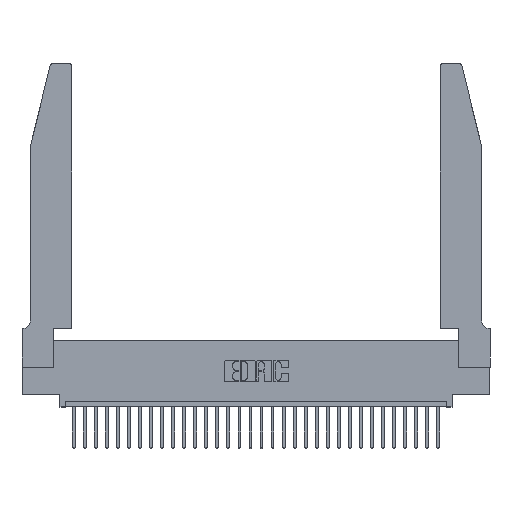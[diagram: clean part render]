
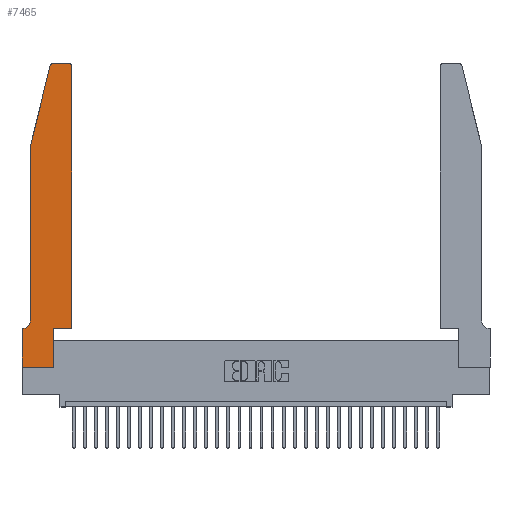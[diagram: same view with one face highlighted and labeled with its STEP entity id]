
A CAD part, top view. The second image highlights one B-rep face of the part: STEP entity #7465.
In plain terms, the highlighted planar face has unit normal (0, 0, 1).
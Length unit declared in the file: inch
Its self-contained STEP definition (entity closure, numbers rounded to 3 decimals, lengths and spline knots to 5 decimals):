
#717 = DIRECTION ( 'NONE',  ( -1., 0., 0. ) ) ;
#1285 = VECTOR ( 'NONE', #17615, 39.37008 ) ;
#1387 = ORIENTED_EDGE ( 'NONE', *, *, #26186, .T. ) ;
#1415 = CARTESIAN_POINT ( 'NONE',  ( 0., 0.35, 0.37 ) ) ;
#1495 = VERTEX_POINT ( 'NONE', #10149 ) ;
#1632 = VECTOR ( 'NONE', #23176, 39.37008 ) ;
#2771 = CARTESIAN_POINT ( 'NONE',  ( 0.2865, 0., 0.37 ) ) ;
#3564 = EDGE_LOOP ( 'NONE', ( #24043, #13470, #21757, #31179, #27198, #29213, #1387, #7926, #9912, #20818, #12689, #25088 ) ) ;
#4615 = CARTESIAN_POINT ( 'NONE',  ( 0.284, 2.72, 0.37 ) ) ;
#4989 = VERTEX_POINT ( 'NONE', #22720 ) ;
#5732 = CARTESIAN_POINT ( 'NONE',  ( 0.4205, 2.75, 0.37 ) ) ;
#5769 = CARTESIAN_POINT ( 'NONE',  ( 0.0755, 0.35, 0.37 ) ) ;
#5818 = CARTESIAN_POINT ( 'NONE',  ( 0.0755, 2., 0.37 ) ) ;
#7255 = DIRECTION ( 'NONE',  ( 1., 0., 0. ) ) ;
#7465 = ADVANCED_FACE ( 'NONE', ( #26915 ), #8958, .T. ) ;
#7489 = DIRECTION ( 'NONE',  ( 1., 0., 0. ) ) ;
#7926 = ORIENTED_EDGE ( 'NONE', *, *, #8728, .T. ) ;
#8214 = CARTESIAN_POINT ( 'NONE',  ( 0.0055, 0.35, 0.37 ) ) ;
#8228 = CARTESIAN_POINT ( 'NONE',  ( 0.4505, 0.35, 0.37 ) ) ;
#8425 = CIRCLE ( 'NONE', #11938, 0.03 ) ;
#8593 = VERTEX_POINT ( 'NONE', #23899 ) ;
#8728 = EDGE_CURVE ( 'NONE', #17757, #23434, #14239, .T. ) ;
#8958 = PLANE ( 'NONE',  #11243 ) ;
#9167 = DIRECTION ( 'NONE',  ( 0., 0., 1. ) ) ;
#9337 = VERTEX_POINT ( 'NONE', #5732 ) ;
#9739 = EDGE_CURVE ( 'NONE', #4989, #26305, #13138, .T. ) ;
#9912 = ORIENTED_EDGE ( 'NONE', *, *, #13290, .T. ) ;
#10149 = CARTESIAN_POINT ( 'NONE',  ( 0.2865, 0.35, 0.37 ) ) ;
#10569 = CIRCLE ( 'NONE', #17640, 0.07 ) ;
#10862 = AXIS2_PLACEMENT_3D ( 'NONE', #4615, #24100, #7489 ) ;
#10893 = CARTESIAN_POINT ( 'NONE',  ( 0.0755, 2., 0.37 ) ) ;
#11243 = AXIS2_PLACEMENT_3D ( 'NONE', #28225, #13633, #7255 ) ;
#11938 = AXIS2_PLACEMENT_3D ( 'NONE', #28125, #9167, #15986 ) ;
#12477 = VECTOR ( 'NONE', #30477, 39.37008 ) ;
#12654 = CARTESIAN_POINT ( 'NONE',  ( 0.4505, 0.35, 0.37 ) ) ;
#12689 = ORIENTED_EDGE ( 'NONE', *, *, #15088, .T. ) ;
#12743 = CARTESIAN_POINT ( 'NONE',  ( 0., 0., 0.37 ) ) ;
#12856 = LINE ( 'NONE', #13256, #21242 ) ;
#12863 = EDGE_CURVE ( 'NONE', #8593, #9337, #8425, .T. ) ;
#13138 = CIRCLE ( 'NONE', #10862, 0.03 ) ;
#13166 = CARTESIAN_POINT ( 'NONE',  ( 0.25487, 2.72718, 0.37 ) ) ;
#13256 = CARTESIAN_POINT ( 'NONE',  ( 0.0755, 2., 0.37 ) ) ;
#13290 = EDGE_CURVE ( 'NONE', #23434, #1495, #16017, .T. ) ;
#13331 = VECTOR ( 'NONE', #25033, 39.37008 ) ;
#13470 = ORIENTED_EDGE ( 'NONE', *, *, #9739, .T. ) ;
#13625 = EDGE_CURVE ( 'NONE', #1495, #31042, #22108, .T. ) ;
#13633 = DIRECTION ( 'NONE',  ( 0., 0., 1. ) ) ;
#13640 = LINE ( 'NONE', #5769, #12477 ) ;
#14239 = LINE ( 'NONE', #15273, #1285 ) ;
#14266 = CARTESIAN_POINT ( 'NONE',  ( 0.0055, 0.42, 0.37 ) ) ;
#15088 = EDGE_CURVE ( 'NONE', #31042, #8593, #31522, .T. ) ;
#15273 = CARTESIAN_POINT ( 'NONE',  ( 0., 0., 0.37 ) ) ;
#15403 = CARTESIAN_POINT ( 'NONE',  ( 0.0755, 0.42, 0.37 ) ) ;
#15986 = DIRECTION ( 'NONE',  ( 1., 0., 0. ) ) ;
#16017 = LINE ( 'NONE', #16853, #25195 ) ;
#16853 = CARTESIAN_POINT ( 'NONE',  ( 0.2865, 0.35, 0.37 ) ) ;
#17342 = EDGE_CURVE ( 'NONE', #29455, #19081, #10569, .T. ) ;
#17615 = DIRECTION ( 'NONE',  ( 1., 0., 0. ) ) ;
#17640 = AXIS2_PLACEMENT_3D ( 'NONE', #14266, #24076, #19473 ) ;
#17749 = DIRECTION ( 'NONE',  ( 0., -1., 0. ) ) ;
#17757 = VERTEX_POINT ( 'NONE', #18494 ) ;
#17840 = CARTESIAN_POINT ( 'NONE',  ( 0.2605, 2.75, 0.37 ) ) ;
#18388 = LINE ( 'NONE', #10893, #1632 ) ;
#18494 = CARTESIAN_POINT ( 'NONE',  ( 0., 0., 0.37 ) ) ;
#19081 = VERTEX_POINT ( 'NONE', #8214 ) ;
#19473 = DIRECTION ( 'NONE',  ( -1., 0., 0. ) ) ;
#19551 = VERTEX_POINT ( 'NONE', #5818 ) ;
#20395 = VERTEX_POINT ( 'NONE', #1415 ) ;
#20818 = ORIENTED_EDGE ( 'NONE', *, *, #13625, .T. ) ;
#21242 = VECTOR ( 'NONE', #25115, 39.37008 ) ;
#21749 = CARTESIAN_POINT ( 'NONE',  ( 0.4505, 0.35, 0.37 ) ) ;
#21757 = ORIENTED_EDGE ( 'NONE', *, *, #27766, .T. ) ;
#22108 = LINE ( 'NONE', #12654, #13331 ) ;
#22720 = CARTESIAN_POINT ( 'NONE',  ( 0.284, 2.75, 0.37 ) ) ;
#23176 = DIRECTION ( 'NONE',  ( 0., -1., 0. ) ) ;
#23434 = VERTEX_POINT ( 'NONE', #2771 ) ;
#23899 = CARTESIAN_POINT ( 'NONE',  ( 0.4505, 2.72, 0.37 ) ) ;
#24043 = ORIENTED_EDGE ( 'NONE', *, *, #29348, .T. ) ;
#24076 = DIRECTION ( 'NONE',  ( 0., 0., -1. ) ) ;
#24100 = DIRECTION ( 'NONE',  ( 0., 0., 1. ) ) ;
#25033 = DIRECTION ( 'NONE',  ( 1., 0., 0. ) ) ;
#25088 = ORIENTED_EDGE ( 'NONE', *, *, #12863, .T. ) ;
#25115 = DIRECTION ( 'NONE',  ( -0.239, -0.971, 0. ) ) ;
#25195 = VECTOR ( 'NONE', #28992, 39.37008 ) ;
#25561 = LINE ( 'NONE', #12743, #30445 ) ;
#26186 = EDGE_CURVE ( 'NONE', #20395, #17757, #25561, .T. ) ;
#26305 = VERTEX_POINT ( 'NONE', #13166 ) ;
#26915 = FACE_OUTER_BOUND ( 'NONE', #3564, .T. ) ;
#27198 = ORIENTED_EDGE ( 'NONE', *, *, #17342, .T. ) ;
#27766 = EDGE_CURVE ( 'NONE', #26305, #19551, #12856, .T. ) ;
#28003 = VECTOR ( 'NONE', #717, 39.37008 ) ;
#28125 = CARTESIAN_POINT ( 'NONE',  ( 0.4205, 2.72, 0.37 ) ) ;
#28225 = CARTESIAN_POINT ( 'NONE',  ( 0., 0.35, 0.37 ) ) ;
#28289 = EDGE_CURVE ( 'NONE', #19081, #20395, #13640, .T. ) ;
#28768 = LINE ( 'NONE', #17840, #28003 ) ;
#28844 = VECTOR ( 'NONE', #30155, 39.37008 ) ;
#28992 = DIRECTION ( 'NONE',  ( 0., 1., 0. ) ) ;
#29213 = ORIENTED_EDGE ( 'NONE', *, *, #28289, .T. ) ;
#29348 = EDGE_CURVE ( 'NONE', #9337, #4989, #28768, .T. ) ;
#29455 = VERTEX_POINT ( 'NONE', #15403 ) ;
#30155 = DIRECTION ( 'NONE',  ( 0., 1., 0. ) ) ;
#30185 = EDGE_CURVE ( 'NONE', #19551, #29455, #18388, .T. ) ;
#30445 = VECTOR ( 'NONE', #17749, 39.37008 ) ;
#30477 = DIRECTION ( 'NONE',  ( -1., 0., 0. ) ) ;
#31042 = VERTEX_POINT ( 'NONE', #21749 ) ;
#31179 = ORIENTED_EDGE ( 'NONE', *, *, #30185, .T. ) ;
#31522 = LINE ( 'NONE', #8228, #28844 ) ;
